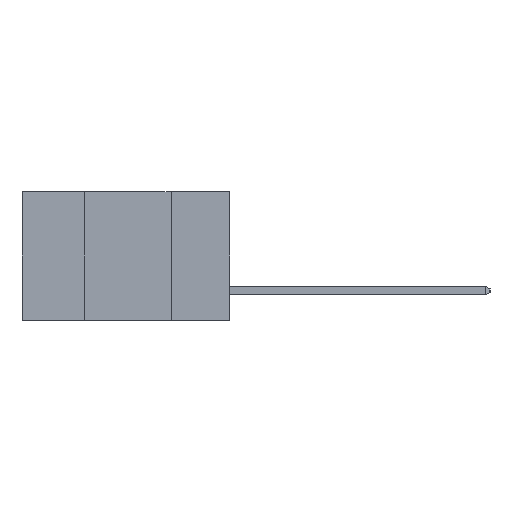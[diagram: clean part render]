
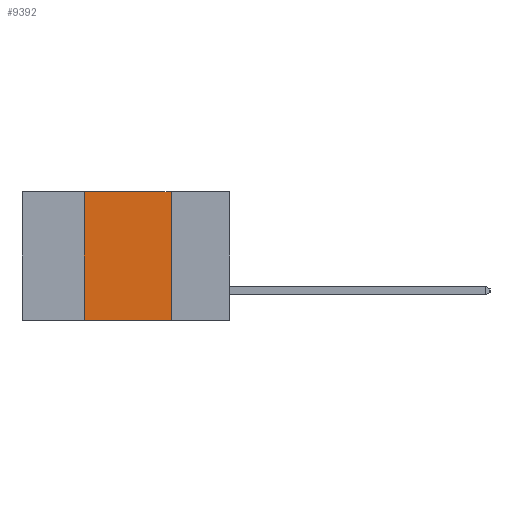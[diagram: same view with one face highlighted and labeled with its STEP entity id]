
A CAD part, left-side view. The second image highlights one B-rep face of the part: STEP entity #9392.
In plain terms, the highlighted planar face has unit normal (-1, 0, 0).
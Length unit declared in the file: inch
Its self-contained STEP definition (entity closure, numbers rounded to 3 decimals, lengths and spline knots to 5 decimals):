
#7 = DIRECTION ( 'NONE',  ( 0., 0., -1. ) ) ;
#47 = EDGE_CURVE ( 'NONE', #7924, #4144, #12165, .T. ) ;
#1625 = EDGE_LOOP ( 'NONE', ( #5963, #2112, #5040, #4637 ) ) ;
#2112 = ORIENTED_EDGE ( 'NONE', *, *, #11771, .F. ) ;
#2369 = DIRECTION ( 'NONE',  ( 0., -1., 0. ) ) ;
#2445 = CARTESIAN_POINT ( 'NONE',  ( 0., 0.6, -0.37 ) ) ;
#2558 = VECTOR ( 'NONE', #2369, 39.37008 ) ;
#2822 = CARTESIAN_POINT ( 'NONE',  ( 0., 0.42, 0. ) ) ;
#4144 = VERTEX_POINT ( 'NONE', #6251 ) ;
#4637 = ORIENTED_EDGE ( 'NONE', *, *, #47, .T. ) ;
#4821 = CARTESIAN_POINT ( 'NONE',  ( 0., 0.42, 0. ) ) ;
#4848 = LINE ( 'NONE', #7523, #9475 ) ;
#5040 = ORIENTED_EDGE ( 'NONE', *, *, #7092, .F. ) ;
#5650 = DIRECTION ( 'NONE',  ( 0., -1., 0. ) ) ;
#5699 = VECTOR ( 'NONE', #9433, 39.37008 ) ;
#5963 = ORIENTED_EDGE ( 'NONE', *, *, #10122, .F. ) ;
#6001 = CARTESIAN_POINT ( 'NONE',  ( 0., 0.17, 0. ) ) ;
#6251 = CARTESIAN_POINT ( 'NONE',  ( 0., 0.17, -0.37 ) ) ;
#6634 = LINE ( 'NONE', #6001, #9096 ) ;
#6787 = DIRECTION ( 'NONE',  ( 0., 0., -1. ) ) ;
#7092 = EDGE_CURVE ( 'NONE', #7924, #8414, #8456, .T. ) ;
#7523 = CARTESIAN_POINT ( 'NONE',  ( 0., 0.6, 0. ) ) ;
#7924 = VERTEX_POINT ( 'NONE', #11445 ) ;
#7991 = FACE_OUTER_BOUND ( 'NONE', #1625, .T. ) ;
#8342 = VERTEX_POINT ( 'NONE', #8435 ) ;
#8414 = VERTEX_POINT ( 'NONE', #2822 ) ;
#8435 = CARTESIAN_POINT ( 'NONE',  ( 0., 0.17, 0. ) ) ;
#8456 = LINE ( 'NONE', #4821, #5699 ) ;
#9096 = VECTOR ( 'NONE', #7, 39.37008 ) ;
#9392 = ADVANCED_FACE ( 'NONE', ( #7991 ), #10413, .F. ) ;
#9433 = DIRECTION ( 'NONE',  ( 0., 0., 1. ) ) ;
#9475 = VECTOR ( 'NONE', #5650, 39.37008 ) ;
#10122 = EDGE_CURVE ( 'NONE', #8342, #4144, #6634, .T. ) ;
#10413 = PLANE ( 'NONE',  #10557 ) ;
#10557 = AXIS2_PLACEMENT_3D ( 'NONE', #11297, #12183, #6787 ) ;
#11297 = CARTESIAN_POINT ( 'NONE',  ( 0., 0.6, 0. ) ) ;
#11445 = CARTESIAN_POINT ( 'NONE',  ( 0., 0.42, -0.37 ) ) ;
#11771 = EDGE_CURVE ( 'NONE', #8414, #8342, #4848, .T. ) ;
#12165 = LINE ( 'NONE', #2445, #2558 ) ;
#12183 = DIRECTION ( 'NONE',  ( 1., 0., 0. ) ) ;
